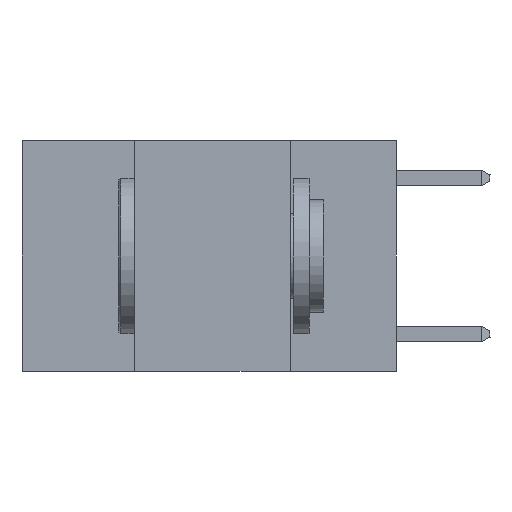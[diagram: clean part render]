
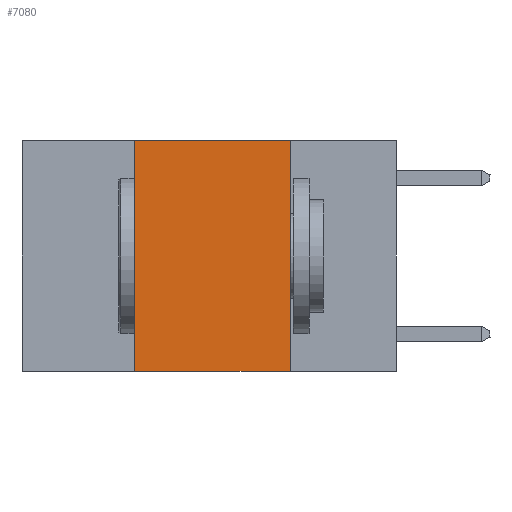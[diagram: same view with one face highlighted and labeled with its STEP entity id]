
A CAD part, left-side view. The second image highlights one B-rep face of the part: STEP entity #7080.
In plain terms, the highlighted planar face has unit normal (-1, 0, 0).
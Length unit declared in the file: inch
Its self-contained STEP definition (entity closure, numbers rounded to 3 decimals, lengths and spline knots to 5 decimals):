
#82 = ORIENTED_EDGE ( 'NONE', *, *, #8658, .F. ) ;
#1772 = VERTEX_POINT ( 'NONE', #16519 ) ;
#2248 = EDGE_CURVE ( 'NONE', #4527, #1772, #9936, .T. ) ;
#2403 = DIRECTION ( 'NONE',  ( 0., 0., -1. ) ) ;
#3715 = FACE_OUTER_BOUND ( 'NONE', #11486, .T. ) ;
#4527 = VERTEX_POINT ( 'NONE', #17482 ) ;
#6118 = CARTESIAN_POINT ( 'NONE',  ( 0., 0.42, 0. ) ) ;
#7080 = ADVANCED_FACE ( 'NONE', ( #3715 ), #14766, .F. ) ;
#7466 = ORIENTED_EDGE ( 'NONE', *, *, #23783, .F. ) ;
#8100 = LINE ( 'NONE', #22702, #16790 ) ;
#8288 = ORIENTED_EDGE ( 'NONE', *, *, #2248, .F. ) ;
#8658 = EDGE_CURVE ( 'NONE', #1772, #22994, #8100, .T. ) ;
#8962 = DIRECTION ( 'NONE',  ( 0., -1., 0. ) ) ;
#9288 = ORIENTED_EDGE ( 'NONE', *, *, #11373, .T. ) ;
#9819 = DIRECTION ( 'NONE',  ( 0., -1., 0. ) ) ;
#9936 = LINE ( 'NONE', #21120, #18145 ) ;
#10259 = VECTOR ( 'NONE', #20954, 39.37008 ) ;
#11026 = CARTESIAN_POINT ( 'NONE',  ( 0., 0.6, -0.37 ) ) ;
#11373 = EDGE_CURVE ( 'NONE', #22821, #22994, #21976, .T. ) ;
#11486 = EDGE_LOOP ( 'NONE', ( #82, #8288, #7466, #9288 ) ) ;
#12587 = CARTESIAN_POINT ( 'NONE',  ( 0., 0.6, 0. ) ) ;
#13631 = LINE ( 'NONE', #6118, #10259 ) ;
#14766 = PLANE ( 'NONE',  #21146 ) ;
#15427 = CARTESIAN_POINT ( 'NONE',  ( 0., 0.42, -0.37 ) ) ;
#16519 = CARTESIAN_POINT ( 'NONE',  ( 0., 0.17, 0. ) ) ;
#16790 = VECTOR ( 'NONE', #2403, 39.37008 ) ;
#17482 = CARTESIAN_POINT ( 'NONE',  ( 0., 0.42, 0. ) ) ;
#18145 = VECTOR ( 'NONE', #9819, 39.37008 ) ;
#19436 = CARTESIAN_POINT ( 'NONE',  ( 0., 0.17, -0.37 ) ) ;
#20954 = DIRECTION ( 'NONE',  ( 0., 0., 1. ) ) ;
#21120 = CARTESIAN_POINT ( 'NONE',  ( 0., 0.6, 0. ) ) ;
#21146 = AXIS2_PLACEMENT_3D ( 'NONE', #12587, #23910, #23776 ) ;
#21976 = LINE ( 'NONE', #11026, #23833 ) ;
#22702 = CARTESIAN_POINT ( 'NONE',  ( 0., 0.17, 0. ) ) ;
#22821 = VERTEX_POINT ( 'NONE', #15427 ) ;
#22994 = VERTEX_POINT ( 'NONE', #19436 ) ;
#23776 = DIRECTION ( 'NONE',  ( 0., 0., -1. ) ) ;
#23783 = EDGE_CURVE ( 'NONE', #22821, #4527, #13631, .T. ) ;
#23833 = VECTOR ( 'NONE', #8962, 39.37008 ) ;
#23910 = DIRECTION ( 'NONE',  ( 1., 0., 0. ) ) ;
